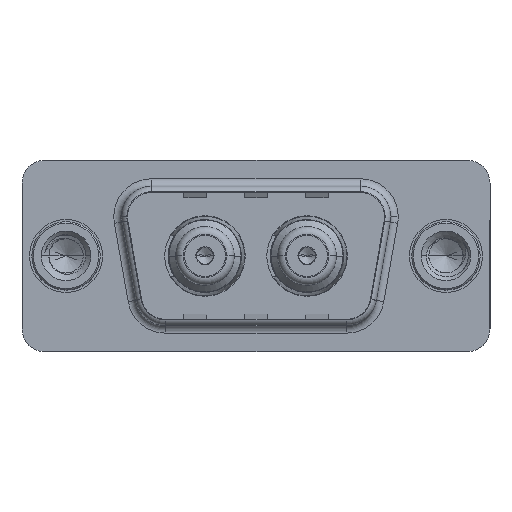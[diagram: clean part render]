
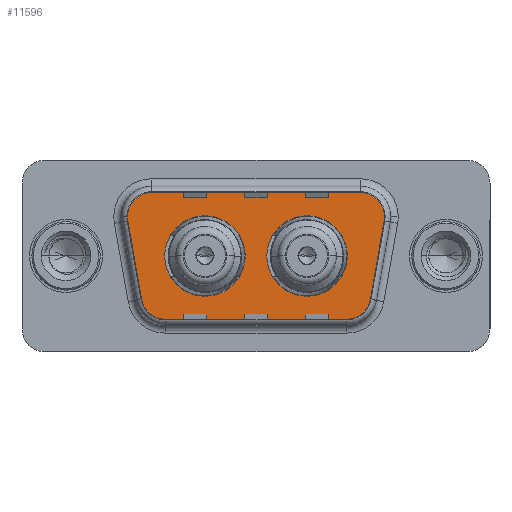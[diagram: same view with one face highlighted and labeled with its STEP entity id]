
A CAD part, top view. The second image highlights one B-rep face of the part: STEP entity #11596.
In plain terms, the highlighted planar face has unit normal (0, 0, 1).
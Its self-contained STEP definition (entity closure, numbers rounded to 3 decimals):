
#132 = CIRCLE ( 'NONE', #11440, 2. ) ;
#266 = ORIENTED_EDGE ( 'NONE', *, *, #7926, .F. ) ;
#349 = CIRCLE ( 'NONE', #6064, 2. ) ;
#568 = EDGE_CURVE ( 'NONE', #19547, #7113, #132, .T. ) ;
#651 = CIRCLE ( 'NONE', #4056, 2.65 ) ;
#663 = CARTESIAN_POINT ( 'NONE',  ( 21.564, 2.9, 0. ) ) ;
#904 = DIRECTION ( 'NONE',  ( 1., 0., 0. ) ) ;
#1166 = EDGE_CURVE ( 'NONE', #20608, #13928, #651, .T. ) ;
#1865 = CIRCLE ( 'NONE', #3157, 2.65 ) ;
#2108 = VERTEX_POINT ( 'NONE', #7942 ) ;
#2412 = VERTEX_POINT ( 'NONE', #5242 ) ;
#2481 = DIRECTION ( 'NONE',  ( 0., 0., 1. ) ) ;
#2516 = AXIS2_PLACEMENT_3D ( 'NONE', #21098, #21072, #21049 ) ;
#2714 = VERTEX_POINT ( 'NONE', #3839 ) ;
#2721 = ORIENTED_EDGE ( 'NONE', *, *, #4662, .T. ) ;
#3060 = CARTESIAN_POINT ( 'NONE',  ( 6.49, 0., 0. ) ) ;
#3157 = AXIS2_PLACEMENT_3D ( 'NONE', #12343, #2481, #13901 ) ;
#3206 = CARTESIAN_POINT ( 'NONE',  ( 18.541, -4.9, 0. ) ) ;
#3839 = CARTESIAN_POINT ( 'NONE',  ( 13.21, 0., 0. ) ) ;
#4056 = AXIS2_PLACEMENT_3D ( 'NONE', #13805, #14347, #5964 ) ;
#4662 = EDGE_CURVE ( 'NONE', #6801, #19547, #7876, .T. ) ;
#4770 = ORIENTED_EDGE ( 'NONE', *, *, #15382, .F. ) ;
#4777 = ORIENTED_EDGE ( 'NONE', *, *, #568, .T. ) ;
#4822 = VERTEX_POINT ( 'NONE', #5639 ) ;
#4865 = EDGE_LOOP ( 'NONE', ( #266, #13758 ) ) ;
#5123 = VERTEX_POINT ( 'NONE', #7460 ) ;
#5242 = CARTESIAN_POINT ( 'NONE',  ( 3.466, 2.553, 0. ) ) ;
#5346 = AXIS2_PLACEMENT_3D ( 'NONE', #15948, #6395, #17560 ) ;
#5379 = CIRCLE ( 'NONE', #17229, 2.65 ) ;
#5578 = LINE ( 'NONE', #18489, #8888 ) ;
#5639 = CARTESIAN_POINT ( 'NONE',  ( 4.489, -3.247, 0. ) ) ;
#5844 = ORIENTED_EDGE ( 'NONE', *, *, #9101, .T. ) ;
#5964 = DIRECTION ( 'NONE',  ( 1., 0., 0. ) ) ;
#6064 = AXIS2_PLACEMENT_3D ( 'NONE', #9769, #21042, #11391 ) ;
#6226 = CARTESIAN_POINT ( 'NONE',  ( 15.86, 0., 0. ) ) ;
#6395 = DIRECTION ( 'NONE',  ( 0., 0., 1. ) ) ;
#6493 = CARTESIAN_POINT ( 'NONE',  ( 20.511, -3.247, 0. ) ) ;
#6510 = PLANE ( 'NONE',  #10007 ) ;
#6702 = CARTESIAN_POINT ( 'NONE',  ( 9.14, 0., 0. ) ) ;
#6801 = VERTEX_POINT ( 'NONE', #9118 ) ;
#7113 = VERTEX_POINT ( 'NONE', #18055 ) ;
#7272 = CARTESIAN_POINT ( 'NONE',  ( 6.459, -4.9, 0. ) ) ;
#7460 = CARTESIAN_POINT ( 'NONE',  ( 5.436, 4.9, 0. ) ) ;
#7869 = DIRECTION ( 'NONE',  ( 1., 0., 0. ) ) ;
#7876 = CIRCLE ( 'NONE', #2516, 2. ) ;
#7926 = EDGE_CURVE ( 'NONE', #13928, #20608, #20289, .T. ) ;
#7942 = CARTESIAN_POINT ( 'NONE',  ( 18.51, 0., 0. ) ) ;
#7990 = CARTESIAN_POINT ( 'NONE',  ( 18.541, -2.9, 0. ) ) ;
#8002 = CIRCLE ( 'NONE', #5346, 2. ) ;
#8123 = DIRECTION ( 'NONE',  ( 0., 0., 1. ) ) ;
#8293 = DIRECTION ( 'NONE',  ( 1., 0., 0. ) ) ;
#8573 = DIRECTION ( 'NONE',  ( -1., 0., 0. ) ) ;
#8888 = VECTOR ( 'NONE', #13921, 1000. ) ;
#8942 = CARTESIAN_POINT ( 'NONE',  ( 6.459, -2.9, 0. ) ) ;
#9101 = EDGE_CURVE ( 'NONE', #5123, #2412, #349, .T. ) ;
#9118 = CARTESIAN_POINT ( 'NONE',  ( 21.534, 2.553, 0. ) ) ;
#9335 = CIRCLE ( 'NONE', #18149, 2. ) ;
#9390 = ORIENTED_EDGE ( 'NONE', *, *, #16033, .F. ) ;
#9529 = LINE ( 'NONE', #12430, #17518 ) ;
#9653 = VERTEX_POINT ( 'NONE', #3206 ) ;
#9720 = DIRECTION ( 'NONE',  ( 0.174, -0.985, 0. ) ) ;
#9769 = CARTESIAN_POINT ( 'NONE',  ( 5.436, 2.9, 0. ) ) ;
#10007 = AXIS2_PLACEMENT_3D ( 'NONE', #7990, #8123, #19306 ) ;
#10055 = FACE_OUTER_BOUND ( 'NONE', #18643, .T. ) ;
#10532 = DIRECTION ( 'NONE',  ( -1., 0., 0. ) ) ;
#10557 = FACE_BOUND ( 'NONE', #18809, .T. ) ;
#10773 = LINE ( 'NONE', #14473, #14451 ) ;
#10866 = EDGE_CURVE ( 'NONE', #7113, #5123, #20122, .T. ) ;
#11391 = DIRECTION ( 'NONE',  ( 1., 0., 0. ) ) ;
#11440 = AXIS2_PLACEMENT_3D ( 'NONE', #15115, #16753, #17026 ) ;
#11596 = ADVANCED_FACE ( 'NONE', ( #10557, #19569, #10055 ), #6510, .T. ) ;
#12320 = EDGE_CURVE ( 'NONE', #18568, #9653, #9529, .T. ) ;
#12343 = CARTESIAN_POINT ( 'NONE',  ( 15.86, 0., 0. ) ) ;
#12346 = AXIS2_PLACEMENT_3D ( 'NONE', #6702, #17854, #8293 ) ;
#12430 = CARTESIAN_POINT ( 'NONE',  ( 6.459, -4.9, 0. ) ) ;
#12561 = EDGE_CURVE ( 'NONE', #2412, #4822, #10773, .T. ) ;
#12759 = ORIENTED_EDGE ( 'NONE', *, *, #13777, .T. ) ;
#12875 = ORIENTED_EDGE ( 'NONE', *, *, #12561, .T. ) ;
#12996 = CARTESIAN_POINT ( 'NONE',  ( 11.79, 0., 0. ) ) ;
#13758 = ORIENTED_EDGE ( 'NONE', *, *, #1166, .F. ) ;
#13777 = EDGE_CURVE ( 'NONE', #9653, #15652, #8002, .T. ) ;
#13805 = CARTESIAN_POINT ( 'NONE',  ( 9.14, 0., 0. ) ) ;
#13901 = DIRECTION ( 'NONE',  ( 1., 0., 0. ) ) ;
#13921 = DIRECTION ( 'NONE',  ( 0.174, 0.985, 0. ) ) ;
#13928 = VERTEX_POINT ( 'NONE', #12996 ) ;
#14347 = DIRECTION ( 'NONE',  ( 0., 0., 1. ) ) ;
#14451 = VECTOR ( 'NONE', #9720, 1000. ) ;
#14473 = CARTESIAN_POINT ( 'NONE',  ( 3.466, 2.553, 0. ) ) ;
#14674 = ORIENTED_EDGE ( 'NONE', *, *, #10866, .T. ) ;
#14833 = ORIENTED_EDGE ( 'NONE', *, *, #17814, .T. ) ;
#15115 = CARTESIAN_POINT ( 'NONE',  ( 19.564, 2.9, 0. ) ) ;
#15382 = EDGE_CURVE ( 'NONE', #2108, #2714, #1865, .T. ) ;
#15652 = VERTEX_POINT ( 'NONE', #6493 ) ;
#15948 = CARTESIAN_POINT ( 'NONE',  ( 18.541, -2.9, 0. ) ) ;
#16033 = EDGE_CURVE ( 'NONE', #2714, #2108, #5379, .T. ) ;
#16753 = DIRECTION ( 'NONE',  ( 0., 0., 1. ) ) ;
#17026 = DIRECTION ( 'NONE',  ( -1., 0., 0. ) ) ;
#17229 = AXIS2_PLACEMENT_3D ( 'NONE', #6226, #17414, #7869 ) ;
#17414 = DIRECTION ( 'NONE',  ( 0., 0., 1. ) ) ;
#17518 = VECTOR ( 'NONE', #904, 1000. ) ;
#17560 = DIRECTION ( 'NONE',  ( 1., 0., 0. ) ) ;
#17814 = EDGE_CURVE ( 'NONE', #15652, #6801, #5578, .T. ) ;
#17854 = DIRECTION ( 'NONE',  ( 0., 0., 1. ) ) ;
#18055 = CARTESIAN_POINT ( 'NONE',  ( 19.564, 4.9, 0. ) ) ;
#18149 = AXIS2_PLACEMENT_3D ( 'NONE', #8942, #20147, #10532 ) ;
#18489 = CARTESIAN_POINT ( 'NONE',  ( 21.534, 2.553, 0. ) ) ;
#18568 = VERTEX_POINT ( 'NONE', #7272 ) ;
#18643 = EDGE_LOOP ( 'NONE', ( #12759, #14833, #2721, #4777, #14674, #5844, #12875, #20013, #19615 ) ) ;
#18809 = EDGE_LOOP ( 'NONE', ( #4770, #9390 ) ) ;
#19306 = DIRECTION ( 'NONE',  ( 1., 0., 0. ) ) ;
#19547 = VERTEX_POINT ( 'NONE', #663 ) ;
#19569 = FACE_BOUND ( 'NONE', #4865, .T. ) ;
#19590 = VECTOR ( 'NONE', #8573, 1000. ) ;
#19615 = ORIENTED_EDGE ( 'NONE', *, *, #12320, .T. ) ;
#19771 = CARTESIAN_POINT ( 'NONE',  ( 5.436, 4.9, 0. ) ) ;
#20013 = ORIENTED_EDGE ( 'NONE', *, *, #20223, .T. ) ;
#20122 = LINE ( 'NONE', #19771, #19590 ) ;
#20147 = DIRECTION ( 'NONE',  ( 0., 0., 1. ) ) ;
#20223 = EDGE_CURVE ( 'NONE', #4822, #18568, #9335, .T. ) ;
#20289 = CIRCLE ( 'NONE', #12346, 2.65 ) ;
#20608 = VERTEX_POINT ( 'NONE', #3060 ) ;
#21042 = DIRECTION ( 'NONE',  ( 0., 0., 1. ) ) ;
#21049 = DIRECTION ( 'NONE',  ( -1., 0., 0. ) ) ;
#21072 = DIRECTION ( 'NONE',  ( 0., 0., 1. ) ) ;
#21098 = CARTESIAN_POINT ( 'NONE',  ( 19.564, 2.9, 0. ) ) ;
